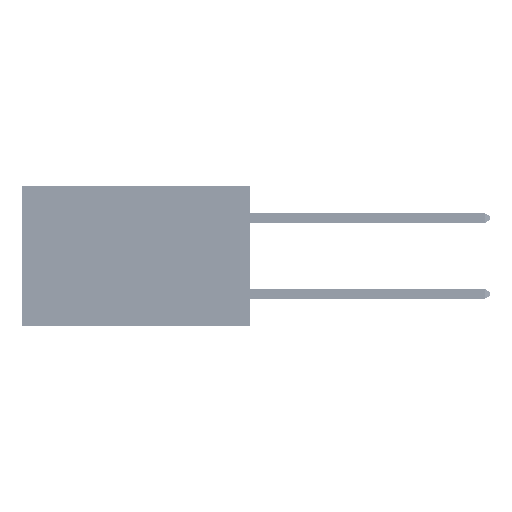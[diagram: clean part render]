
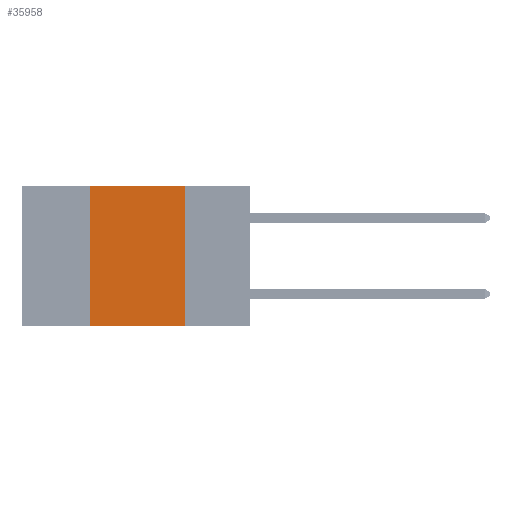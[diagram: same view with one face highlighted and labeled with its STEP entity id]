
A CAD part, left-side view. The second image highlights one B-rep face of the part: STEP entity #35958.
In plain terms, the highlighted planar face has unit normal (-1, 0, 0).
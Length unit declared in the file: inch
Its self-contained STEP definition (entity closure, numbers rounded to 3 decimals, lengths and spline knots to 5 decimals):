
#1987 = AXIS2_PLACEMENT_3D ( 'NONE', #34886, #26568, #14444 ) ;
#2952 = LINE ( 'NONE', #33965, #34068 ) ;
#3476 = VECTOR ( 'NONE', #42338, 39.37008 ) ;
#7068 = CARTESIAN_POINT ( 'NONE',  ( 0., 0.42, 0. ) ) ;
#7685 = ORIENTED_EDGE ( 'NONE', *, *, #26423, .F. ) ;
#9645 = DIRECTION ( 'NONE',  ( 0., -1., 0. ) ) ;
#11273 = ORIENTED_EDGE ( 'NONE', *, *, #36580, .T. ) ;
#13375 = DIRECTION ( 'NONE',  ( 0., 0., -1. ) ) ;
#14444 = DIRECTION ( 'NONE',  ( 0., 0., -1. ) ) ;
#17261 = ORIENTED_EDGE ( 'NONE', *, *, #21421, .F. ) ;
#17972 = EDGE_LOOP ( 'NONE', ( #19997, #7685, #17261, #11273 ) ) ;
#19997 = ORIENTED_EDGE ( 'NONE', *, *, #45627, .F. ) ;
#21421 = EDGE_CURVE ( 'NONE', #25286, #32941, #22971, .T. ) ;
#22971 = LINE ( 'NONE', #33822, #3476 ) ;
#23058 = FACE_OUTER_BOUND ( 'NONE', #17972, .T. ) ;
#23289 = VERTEX_POINT ( 'NONE', #39861 ) ;
#24039 = LINE ( 'NONE', #46588, #26616 ) ;
#25286 = VERTEX_POINT ( 'NONE', #30830 ) ;
#26423 = EDGE_CURVE ( 'NONE', #32941, #31794, #2952, .T. ) ;
#26568 = DIRECTION ( 'NONE',  ( 1., 0., 0. ) ) ;
#26616 = VECTOR ( 'NONE', #13375, 39.37008 ) ;
#30830 = CARTESIAN_POINT ( 'NONE',  ( 0., 0.42, -0.37 ) ) ;
#31794 = VERTEX_POINT ( 'NONE', #37953 ) ;
#32941 = VERTEX_POINT ( 'NONE', #7068 ) ;
#33822 = CARTESIAN_POINT ( 'NONE',  ( 0., 0.42, 0. ) ) ;
#33965 = CARTESIAN_POINT ( 'NONE',  ( 0., 0.6, 0. ) ) ;
#34068 = VECTOR ( 'NONE', #46514, 39.37008 ) ;
#34886 = CARTESIAN_POINT ( 'NONE',  ( 0., 0.6, 0. ) ) ;
#35958 = ADVANCED_FACE ( 'NONE', ( #23058 ), #39251, .F. ) ;
#36580 = EDGE_CURVE ( 'NONE', #25286, #23289, #42707, .T. ) ;
#37491 = VECTOR ( 'NONE', #9645, 39.37008 ) ;
#37953 = CARTESIAN_POINT ( 'NONE',  ( 0., 0.17, 0. ) ) ;
#38473 = CARTESIAN_POINT ( 'NONE',  ( 0., 0.6, -0.37 ) ) ;
#39251 = PLANE ( 'NONE',  #1987 ) ;
#39861 = CARTESIAN_POINT ( 'NONE',  ( 0., 0.17, -0.37 ) ) ;
#42338 = DIRECTION ( 'NONE',  ( 0., 0., 1. ) ) ;
#42707 = LINE ( 'NONE', #38473, #37491 ) ;
#45627 = EDGE_CURVE ( 'NONE', #31794, #23289, #24039, .T. ) ;
#46514 = DIRECTION ( 'NONE',  ( 0., -1., 0. ) ) ;
#46588 = CARTESIAN_POINT ( 'NONE',  ( 0., 0.17, 0. ) ) ;
